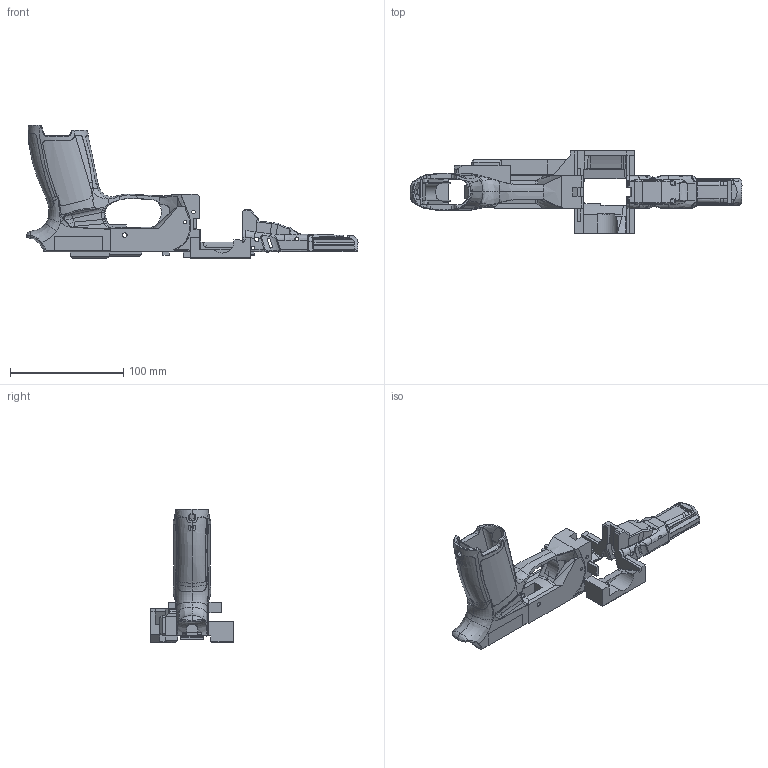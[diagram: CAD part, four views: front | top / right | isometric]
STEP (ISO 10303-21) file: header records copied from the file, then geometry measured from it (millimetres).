
FILE_DESCRIPTION(/* description */ (''),/* implementation_level */ '2;1');
FILE_NAME(/* name */ '',/* time_stamp */ '',/* author */ (''),/* organization */ (''),/* preprocessor_version */ 'ST-DEVELOPER v18',/* originating_system */ '',/* authorisation */ '');
FILE_SCHEMA (('AUTOMOTIVE_DESIGN { 1 0 10303 214 3 1 1 }'));
Products named in the file (4): Assembly31; Glockoma Vityaz's Folly ALPHA; Tigger bar v6.3; mag catch block 3mm
Assembly tree (2 placements, depth 2):
  Assembly31
    Tigger bar v6.3
    mag catch block 3mm
  Glockoma Vityaz's Folly ALPHA
Bounding box: 293.23 x 73.17 x 117.8 mm (x, y, z)
Volume: 199424.7 mm3; surface area: 87372.5 mm2
Topology: 6 solids, 10 shells, 1326 faces, 3632 edges, 2288 vertices
Faces by surface type: plane 603, bspline 402, cylinder 261, torus 31, cone 15, sphere 14
Full cylindrical faces by diameter (mm): 3 x4, 3.2 x2, 3.302 x2, 4 x4
Entity records: 85119 total; most frequent: CARTESIAN_POINT 54048, ORIENTED_EDGE 7236, DIRECTION 5384, EDGE_CURVE 3618, VERTEX_POINT 2288, LINE 1888, VECTOR 1888, AXIS2_PLACEMENT_3D 1748
